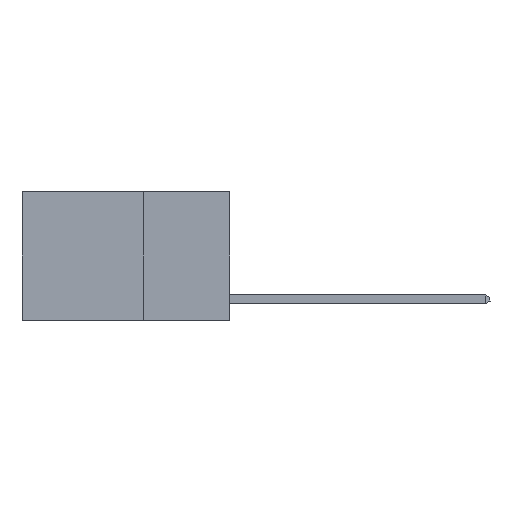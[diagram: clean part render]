
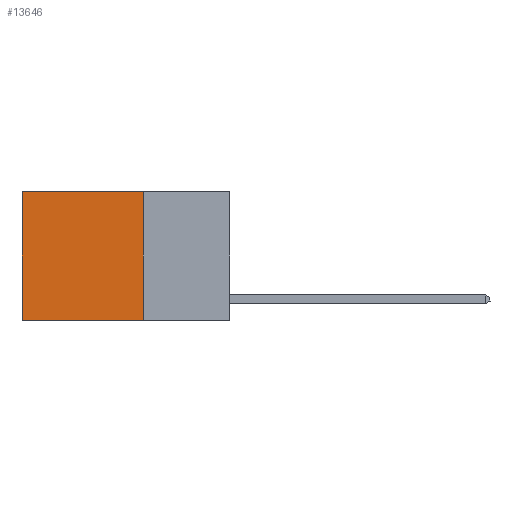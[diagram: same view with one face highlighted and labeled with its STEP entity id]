
A CAD part, left-side view. The second image highlights one B-rep face of the part: STEP entity #13646.
In plain terms, the highlighted planar face has unit normal (-1, 0, 0).
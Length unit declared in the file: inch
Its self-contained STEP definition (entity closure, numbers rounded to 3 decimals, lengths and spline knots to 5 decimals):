
#266 = VERTEX_POINT ( 'NONE', #14657 ) ;
#344 = VERTEX_POINT ( 'NONE', #7431 ) ;
#1866 = EDGE_CURVE ( 'NONE', #16008, #266, #3165, .T. ) ;
#3165 = LINE ( 'NONE', #9905, #16972 ) ;
#3910 = CARTESIAN_POINT ( 'NONE',  ( 0.2625, 0.25, 0. ) ) ;
#4958 = LINE ( 'NONE', #23568, #9386 ) ;
#7220 = VECTOR ( 'NONE', #17043, 39.37008 ) ;
#7431 = CARTESIAN_POINT ( 'NONE',  ( 0.2625, 0.25, -0.37 ) ) ;
#9381 = FACE_OUTER_BOUND ( 'NONE', #15836, .T. ) ;
#9386 = VECTOR ( 'NONE', #16253, 39.37008 ) ;
#9905 = CARTESIAN_POINT ( 'NONE',  ( 0.2625, 0.6, 0. ) ) ;
#10541 = CARTESIAN_POINT ( 'NONE',  ( 0.2625, 0.6, 0. ) ) ;
#11340 = AXIS2_PLACEMENT_3D ( 'NONE', #16985, #22507, #11437 ) ;
#11437 = DIRECTION ( 'NONE',  ( 0., 0., -1. ) ) ;
#12111 = EDGE_CURVE ( 'NONE', #344, #266, #19984, .T. ) ;
#12814 = LINE ( 'NONE', #3910, #7220 ) ;
#13646 = ADVANCED_FACE ( 'NONE', ( #9381 ), #20688, .F. ) ;
#13918 = VECTOR ( 'NONE', #16230, 39.37008 ) ;
#14248 = VERTEX_POINT ( 'NONE', #19563 ) ;
#14399 = CARTESIAN_POINT ( 'NONE',  ( 0.2625, 0.25, -0.37 ) ) ;
#14657 = CARTESIAN_POINT ( 'NONE',  ( 0.2625, 0.6, -0.37 ) ) ;
#15339 = ORIENTED_EDGE ( 'NONE', *, *, #21659, .F. ) ;
#15836 = EDGE_LOOP ( 'NONE', ( #19086, #21151, #15339, #22982 ) ) ;
#16008 = VERTEX_POINT ( 'NONE', #10541 ) ;
#16230 = DIRECTION ( 'NONE',  ( 0., 1., 0. ) ) ;
#16253 = DIRECTION ( 'NONE',  ( 0., 1., 0. ) ) ;
#16972 = VECTOR ( 'NONE', #19191, 39.37008 ) ;
#16985 = CARTESIAN_POINT ( 'NONE',  ( 0.2625, 0.25, 0. ) ) ;
#17043 = DIRECTION ( 'NONE',  ( 0., 0., -1. ) ) ;
#19086 = ORIENTED_EDGE ( 'NONE', *, *, #1866, .T. ) ;
#19191 = DIRECTION ( 'NONE',  ( 0., 0., -1. ) ) ;
#19563 = CARTESIAN_POINT ( 'NONE',  ( 0.2625, 0.25, 0. ) ) ;
#19984 = LINE ( 'NONE', #14399, #13918 ) ;
#20688 = PLANE ( 'NONE',  #11340 ) ;
#20803 = EDGE_CURVE ( 'NONE', #14248, #16008, #4958, .T. ) ;
#21151 = ORIENTED_EDGE ( 'NONE', *, *, #12111, .F. ) ;
#21659 = EDGE_CURVE ( 'NONE', #14248, #344, #12814, .T. ) ;
#22507 = DIRECTION ( 'NONE',  ( 1., 0., 0. ) ) ;
#22982 = ORIENTED_EDGE ( 'NONE', *, *, #20803, .T. ) ;
#23568 = CARTESIAN_POINT ( 'NONE',  ( 0.2625, 0.25, 0. ) ) ;
